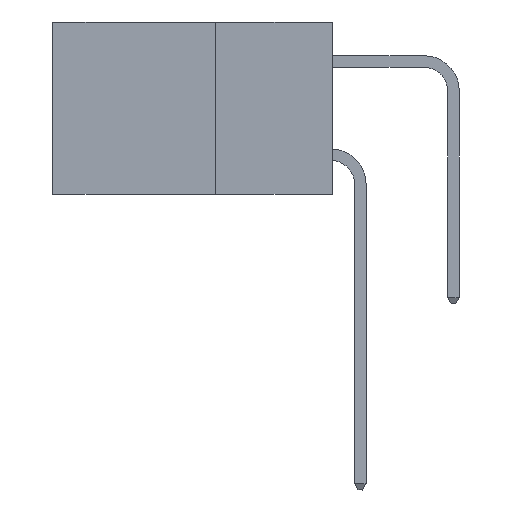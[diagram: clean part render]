
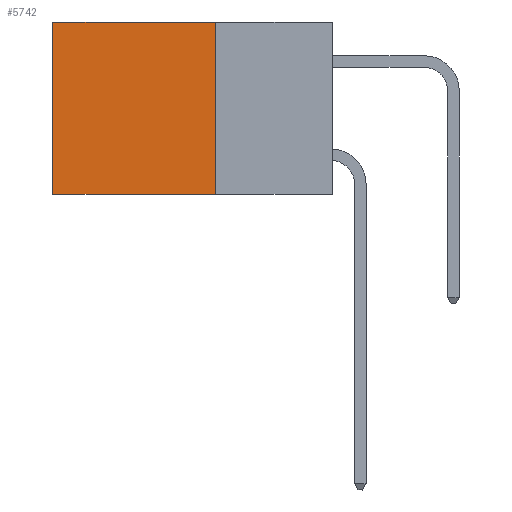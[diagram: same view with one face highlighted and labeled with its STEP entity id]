
A CAD part, left-side view. The second image highlights one B-rep face of the part: STEP entity #5742.
In plain terms, the highlighted planar face has unit normal (-1, 0, 0).
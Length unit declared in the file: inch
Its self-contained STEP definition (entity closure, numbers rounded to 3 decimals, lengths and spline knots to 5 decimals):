
#288 = CARTESIAN_POINT ( 'NONE',  ( 0.298, 0.25, 0. ) ) ;
#706 = LINE ( 'NONE', #15592, #13707 ) ;
#1075 = VECTOR ( 'NONE', #12953, 39.37008 ) ;
#1246 = EDGE_CURVE ( 'NONE', #4796, #9283, #4896, .T. ) ;
#1312 = CARTESIAN_POINT ( 'NONE',  ( 0.298, 0.25, 0. ) ) ;
#1909 = DIRECTION ( 'NONE',  ( 0., 0., -1. ) ) ;
#2043 = ORIENTED_EDGE ( 'NONE', *, *, #1246, .T. ) ;
#3432 = AXIS2_PLACEMENT_3D ( 'NONE', #7034, #6825, #6800 ) ;
#4200 = CARTESIAN_POINT ( 'NONE',  ( 0.298, 0.6, 0. ) ) ;
#4796 = VERTEX_POINT ( 'NONE', #4200 ) ;
#4896 = LINE ( 'NONE', #11513, #11334 ) ;
#5536 = DIRECTION ( 'NONE',  ( 0., 1., 0. ) ) ;
#5742 = ADVANCED_FACE ( 'NONE', ( #15961 ), #7088, .F. ) ;
#6800 = DIRECTION ( 'NONE',  ( 0., 0., -1. ) ) ;
#6825 = DIRECTION ( 'NONE',  ( 1., 0., 0. ) ) ;
#7034 = CARTESIAN_POINT ( 'NONE',  ( 0.298, 0.25, 0. ) ) ;
#7088 = PLANE ( 'NONE',  #3432 ) ;
#7558 = EDGE_LOOP ( 'NONE', ( #2043, #12300, #9176, #15113 ) ) ;
#7585 = VERTEX_POINT ( 'NONE', #7690 ) ;
#7690 = CARTESIAN_POINT ( 'NONE',  ( 0.298, 0.25, -0.37 ) ) ;
#7707 = LINE ( 'NONE', #288, #1075 ) ;
#8325 = DIRECTION ( 'NONE',  ( 0., 0., -1. ) ) ;
#8330 = VECTOR ( 'NONE', #8325, 39.37008 ) ;
#8851 = CARTESIAN_POINT ( 'NONE',  ( 0.298, 0.6, -0.37 ) ) ;
#9176 = ORIENTED_EDGE ( 'NONE', *, *, #12162, .F. ) ;
#9283 = VERTEX_POINT ( 'NONE', #8851 ) ;
#10547 = LINE ( 'NONE', #12279, #8330 ) ;
#11334 = VECTOR ( 'NONE', #1909, 39.37008 ) ;
#11513 = CARTESIAN_POINT ( 'NONE',  ( 0.298, 0.6, 0. ) ) ;
#12162 = EDGE_CURVE ( 'NONE', #14951, #7585, #10547, .T. ) ;
#12279 = CARTESIAN_POINT ( 'NONE',  ( 0.298, 0.25, 0. ) ) ;
#12300 = ORIENTED_EDGE ( 'NONE', *, *, #13975, .F. ) ;
#12953 = DIRECTION ( 'NONE',  ( 0., 1., 0. ) ) ;
#13707 = VECTOR ( 'NONE', #5536, 39.37008 ) ;
#13975 = EDGE_CURVE ( 'NONE', #7585, #9283, #706, .T. ) ;
#14349 = EDGE_CURVE ( 'NONE', #14951, #4796, #7707, .T. ) ;
#14951 = VERTEX_POINT ( 'NONE', #1312 ) ;
#15113 = ORIENTED_EDGE ( 'NONE', *, *, #14349, .T. ) ;
#15592 = CARTESIAN_POINT ( 'NONE',  ( 0.298, 0.25, -0.37 ) ) ;
#15961 = FACE_OUTER_BOUND ( 'NONE', #7558, .T. ) ;
